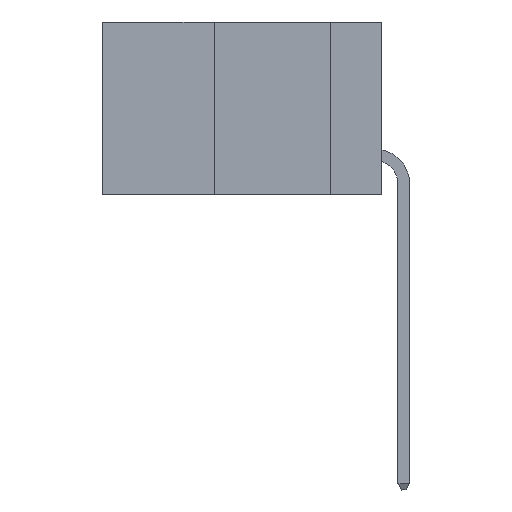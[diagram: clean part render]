
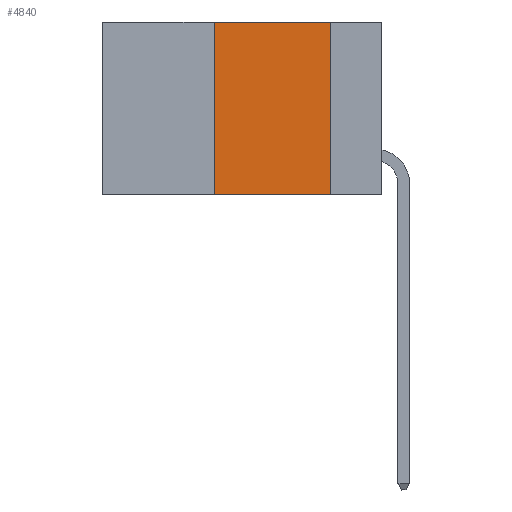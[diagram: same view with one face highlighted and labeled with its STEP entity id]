
A CAD part, left-side view. The second image highlights one B-rep face of the part: STEP entity #4840.
In plain terms, the highlighted planar face has unit normal (-1, 0, 0).
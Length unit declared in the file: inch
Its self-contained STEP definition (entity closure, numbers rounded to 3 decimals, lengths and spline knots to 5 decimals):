
#1 = LINE ( 'NONE', #20676, #5529 ) ;
#919 = AXIS2_PLACEMENT_3D ( 'NONE', #11209, #24325, #14787 ) ;
#939 = VECTOR ( 'NONE', #22786, 39.37008 ) ;
#2333 = VERTEX_POINT ( 'NONE', #23683 ) ;
#2984 = DIRECTION ( 'NONE',  ( 0., 0., 1. ) ) ;
#3170 = VERTEX_POINT ( 'NONE', #22222 ) ;
#3518 = DIRECTION ( 'NONE',  ( 0., -1., 0. ) ) ;
#4212 = CARTESIAN_POINT ( 'NONE',  ( 0., 0.6, -0.37 ) ) ;
#4369 = EDGE_CURVE ( 'NONE', #16308, #3170, #1, .T. ) ;
#4840 = ADVANCED_FACE ( 'NONE', ( #7830 ), #7313, .F. ) ;
#5194 = ORIENTED_EDGE ( 'NONE', *, *, #14645, .F. ) ;
#5225 = CARTESIAN_POINT ( 'NONE',  ( 0., 0.6, 0. ) ) ;
#5529 = VECTOR ( 'NONE', #19472, 39.37008 ) ;
#5830 = CARTESIAN_POINT ( 'NONE',  ( 0., 0.36, -0.37 ) ) ;
#6445 = EDGE_CURVE ( 'NONE', #2333, #16308, #19243, .T. ) ;
#7313 = PLANE ( 'NONE',  #919 ) ;
#7830 = FACE_OUTER_BOUND ( 'NONE', #10928, .T. ) ;
#7891 = VECTOR ( 'NONE', #2984, 39.37008 ) ;
#10928 = EDGE_LOOP ( 'NONE', ( #21123, #17800, #5194, #17790 ) ) ;
#11209 = CARTESIAN_POINT ( 'NONE',  ( 0., 0.6, 0. ) ) ;
#12740 = VERTEX_POINT ( 'NONE', #5830 ) ;
#14285 = CARTESIAN_POINT ( 'NONE',  ( 0., 0.36, 0. ) ) ;
#14444 = LINE ( 'NONE', #14285, #7891 ) ;
#14645 = EDGE_CURVE ( 'NONE', #12740, #2333, #14444, .T. ) ;
#14787 = DIRECTION ( 'NONE',  ( 0., 0., -1. ) ) ;
#16308 = VERTEX_POINT ( 'NONE', #23485 ) ;
#17790 = ORIENTED_EDGE ( 'NONE', *, *, #18965, .T. ) ;
#17791 = VECTOR ( 'NONE', #3518, 39.37008 ) ;
#17800 = ORIENTED_EDGE ( 'NONE', *, *, #6445, .F. ) ;
#18965 = EDGE_CURVE ( 'NONE', #12740, #3170, #20363, .T. ) ;
#19243 = LINE ( 'NONE', #5225, #17791 ) ;
#19472 = DIRECTION ( 'NONE',  ( 0., 0., -1. ) ) ;
#20363 = LINE ( 'NONE', #4212, #939 ) ;
#20676 = CARTESIAN_POINT ( 'NONE',  ( 0., 0.11, 0. ) ) ;
#21123 = ORIENTED_EDGE ( 'NONE', *, *, #4369, .F. ) ;
#22222 = CARTESIAN_POINT ( 'NONE',  ( 0., 0.11, -0.37 ) ) ;
#22786 = DIRECTION ( 'NONE',  ( 0., -1., 0. ) ) ;
#23485 = CARTESIAN_POINT ( 'NONE',  ( 0., 0.11, 0. ) ) ;
#23683 = CARTESIAN_POINT ( 'NONE',  ( 0., 0.36, 0. ) ) ;
#24325 = DIRECTION ( 'NONE',  ( 1., 0., 0. ) ) ;
